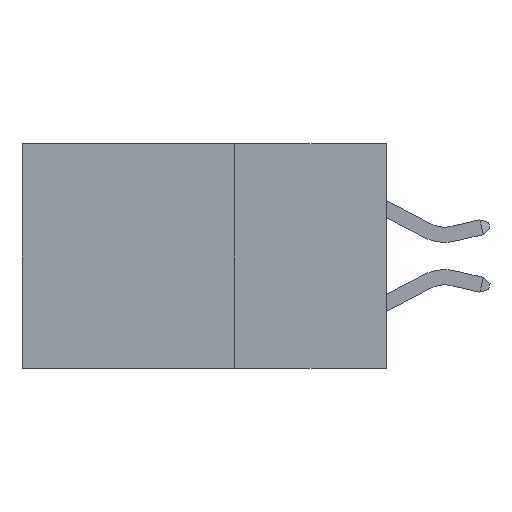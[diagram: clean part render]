
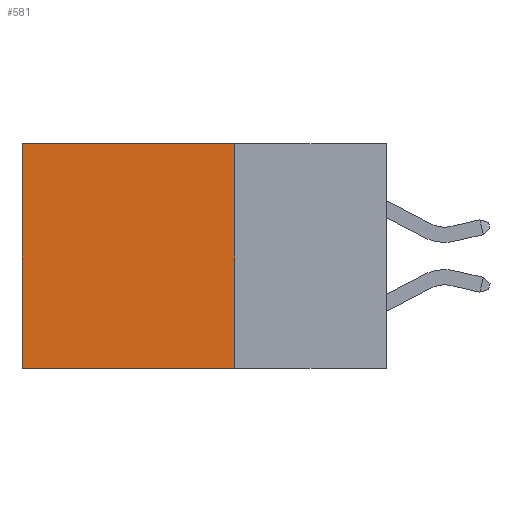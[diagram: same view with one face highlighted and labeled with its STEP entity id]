
A CAD part, left-side view. The second image highlights one B-rep face of the part: STEP entity #581.
In plain terms, the highlighted planar face has unit normal (-1, 0, 0).
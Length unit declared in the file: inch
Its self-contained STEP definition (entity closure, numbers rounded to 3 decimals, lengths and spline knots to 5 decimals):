
#59 = ORIENTED_EDGE ( 'NONE', *, *, #1376, .F. ) ;
#581 = ADVANCED_FACE ( 'NONE', ( #8807 ), #13190, .F. ) ;
#1376 = EDGE_CURVE ( 'NONE', #14284, #6099, #1678, .T. ) ;
#1678 = LINE ( 'NONE', #11102, #13141 ) ;
#1816 = CARTESIAN_POINT ( 'NONE',  ( 0.2615, 0.6, 0. ) ) ;
#1840 = DIRECTION ( 'NONE',  ( 0., 1., 0. ) ) ;
#2050 = CARTESIAN_POINT ( 'NONE',  ( 0.2615, 0.25, 0. ) ) ;
#3497 = DIRECTION ( 'NONE',  ( 0., 0., -1. ) ) ;
#3549 = CARTESIAN_POINT ( 'NONE',  ( 0.2615, 0.25, 0. ) ) ;
#3554 = CARTESIAN_POINT ( 'NONE',  ( 0.2615, 0.6, -0.37 ) ) ;
#3903 = DIRECTION ( 'NONE',  ( 0., 0., -1. ) ) ;
#3915 = CARTESIAN_POINT ( 'NONE',  ( 0.2615, 0.6, -0.37 ) ) ;
#4237 = EDGE_CURVE ( 'NONE', #14284, #6488, #13043, .T. ) ;
#4264 = CARTESIAN_POINT ( 'NONE',  ( 0.2615, 0.25, -0.37 ) ) ;
#4439 = VECTOR ( 'NONE', #1840, 39.37008 ) ;
#4953 = CARTESIAN_POINT ( 'NONE',  ( 0.2615, 0.25, -0.37 ) ) ;
#5053 = EDGE_CURVE ( 'NONE', #6099, #9344, #13800, .T. ) ;
#6099 = VERTEX_POINT ( 'NONE', #4953 ) ;
#6488 = VERTEX_POINT ( 'NONE', #1816 ) ;
#7870 = ORIENTED_EDGE ( 'NONE', *, *, #5053, .F. ) ;
#8003 = VECTOR ( 'NONE', #13021, 39.37008 ) ;
#8483 = LINE ( 'NONE', #3915, #11955 ) ;
#8807 = FACE_OUTER_BOUND ( 'NONE', #12181, .T. ) ;
#9344 = VERTEX_POINT ( 'NONE', #3554 ) ;
#9720 = EDGE_CURVE ( 'NONE', #6488, #9344, #8483, .T. ) ;
#10113 = DIRECTION ( 'NONE',  ( 1., 0., 0. ) ) ;
#11102 = CARTESIAN_POINT ( 'NONE',  ( 0.2615, 0.25, -0.37 ) ) ;
#11130 = DIRECTION ( 'NONE',  ( 0., 0., -1. ) ) ;
#11955 = VECTOR ( 'NONE', #3903, 39.37008 ) ;
#12181 = EDGE_LOOP ( 'NONE', ( #13645, #7870, #59, #13522 ) ) ;
#12973 = AXIS2_PLACEMENT_3D ( 'NONE', #4264, #10113, #3497 ) ;
#13021 = DIRECTION ( 'NONE',  ( 0., 1., 0. ) ) ;
#13043 = LINE ( 'NONE', #2050, #4439 ) ;
#13115 = CARTESIAN_POINT ( 'NONE',  ( 0.2615, 0.25, -0.37 ) ) ;
#13141 = VECTOR ( 'NONE', #11130, 39.37008 ) ;
#13190 = PLANE ( 'NONE',  #12973 ) ;
#13522 = ORIENTED_EDGE ( 'NONE', *, *, #4237, .T. ) ;
#13645 = ORIENTED_EDGE ( 'NONE', *, *, #9720, .T. ) ;
#13800 = LINE ( 'NONE', #13115, #8003 ) ;
#14284 = VERTEX_POINT ( 'NONE', #3549 ) ;
